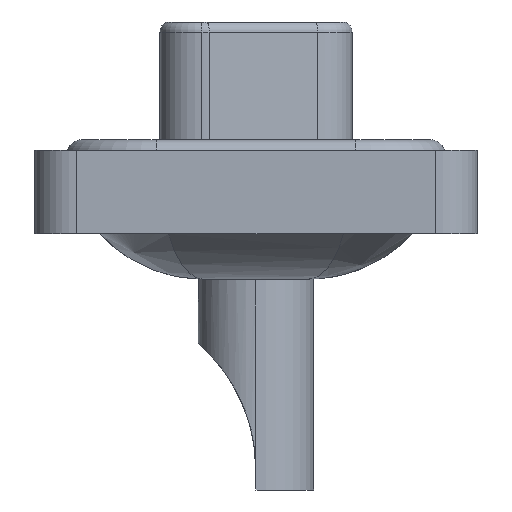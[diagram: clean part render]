
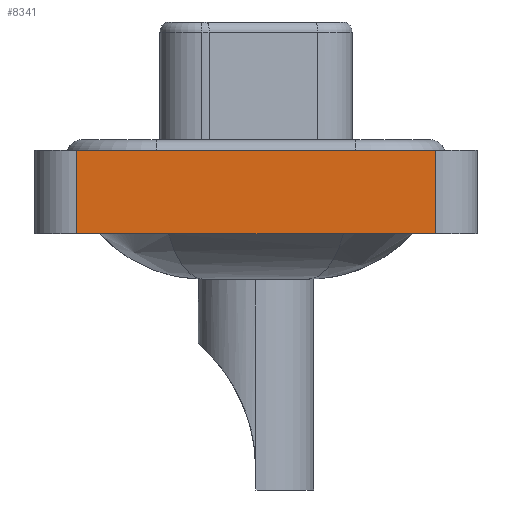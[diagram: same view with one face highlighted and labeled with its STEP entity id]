
A CAD part, left-side view. The second image highlights one B-rep face of the part: STEP entity #8341.
In plain terms, the highlighted planar face has unit normal (-1, 0, 0).
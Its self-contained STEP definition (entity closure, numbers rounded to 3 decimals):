
#149 = DIRECTION ( 'NONE',  ( 0., 0., 1. ) ) ;
#173 = VECTOR ( 'NONE', #149, 1000. ) ;
#346 = ORIENTED_EDGE ( 'NONE', *, *, #15703, .F. ) ;
#906 = DIRECTION ( 'NONE',  ( 0., 0., 1. ) ) ;
#1444 = CARTESIAN_POINT ( 'NONE',  ( -7.3, 8.55, 0.4 ) ) ;
#2918 = LINE ( 'NONE', #4093, #16108 ) ;
#2958 = CARTESIAN_POINT ( 'NONE',  ( -7.3, 8.55, -3.6 ) ) ;
#3024 = DIRECTION ( 'NONE',  ( 0., -1., 0. ) ) ;
#3379 = EDGE_CURVE ( 'NONE', #7164, #10818, #2918, .T. ) ;
#3606 = CARTESIAN_POINT ( 'NONE',  ( -7.3, -8.55, -3.6 ) ) ;
#4093 = CARTESIAN_POINT ( 'NONE',  ( -7.3, -8.55, -3.6 ) ) ;
#4135 = CARTESIAN_POINT ( 'NONE',  ( -7.3, -8.55, 0.4 ) ) ;
#4338 = DIRECTION ( 'NONE',  ( 0., -1., 0. ) ) ;
#4630 = LINE ( 'NONE', #4720, #7995 ) ;
#4720 = CARTESIAN_POINT ( 'NONE',  ( -7.3, -8.55, -3.6 ) ) ;
#5474 = CARTESIAN_POINT ( 'NONE',  ( -7.3, -8.55, 0.4 ) ) ;
#5512 = CARTESIAN_POINT ( 'NONE',  ( -7.3, -8.55, -3.6 ) ) ;
#6563 = AXIS2_PLACEMENT_3D ( 'NONE', #3606, #10096, #15305 ) ;
#7164 = VERTEX_POINT ( 'NONE', #9386 ) ;
#7380 = VERTEX_POINT ( 'NONE', #1444 ) ;
#7995 = VECTOR ( 'NONE', #906, 1000. ) ;
#8341 = ADVANCED_FACE ( 'NONE', ( #15639 ), #14280, .T. ) ;
#8739 = ORIENTED_EDGE ( 'NONE', *, *, #9542, .T. ) ;
#9272 = LINE ( 'NONE', #4135, #14584 ) ;
#9386 = CARTESIAN_POINT ( 'NONE',  ( -7.3, 8.55, -3.6 ) ) ;
#9408 = ORIENTED_EDGE ( 'NONE', *, *, #11754, .F. ) ;
#9542 = EDGE_CURVE ( 'NONE', #10818, #11889, #4630, .T. ) ;
#10096 = DIRECTION ( 'NONE',  ( -1., 0., 0. ) ) ;
#10818 = VERTEX_POINT ( 'NONE', #5512 ) ;
#11754 = EDGE_CURVE ( 'NONE', #7164, #7380, #15836, .T. ) ;
#11889 = VERTEX_POINT ( 'NONE', #5474 ) ;
#13779 = EDGE_LOOP ( 'NONE', ( #8739, #346, #9408, #16096 ) ) ;
#14280 = PLANE ( 'NONE',  #6563 ) ;
#14584 = VECTOR ( 'NONE', #3024, 1000. ) ;
#15305 = DIRECTION ( 'NONE',  ( 0., 0., 1. ) ) ;
#15639 = FACE_OUTER_BOUND ( 'NONE', #13779, .T. ) ;
#15703 = EDGE_CURVE ( 'NONE', #7380, #11889, #9272, .T. ) ;
#15836 = LINE ( 'NONE', #2958, #173 ) ;
#16096 = ORIENTED_EDGE ( 'NONE', *, *, #3379, .T. ) ;
#16108 = VECTOR ( 'NONE', #4338, 1000. ) ;
